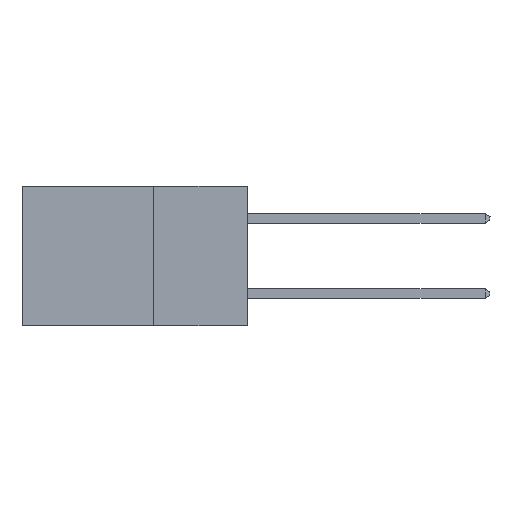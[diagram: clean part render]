
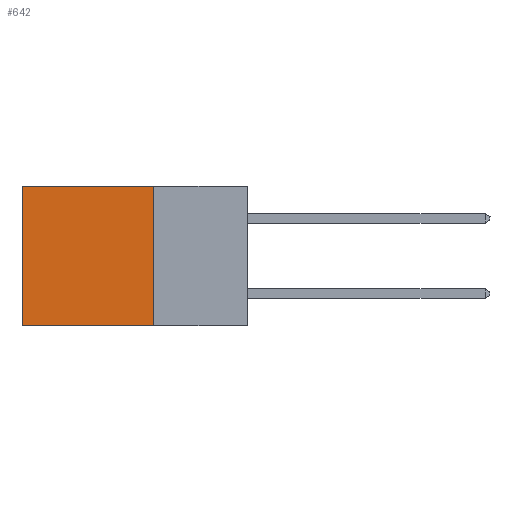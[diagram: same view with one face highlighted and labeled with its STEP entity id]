
A CAD part, left-side view. The second image highlights one B-rep face of the part: STEP entity #642.
In plain terms, the highlighted planar face has unit normal (-1, 0, 0).
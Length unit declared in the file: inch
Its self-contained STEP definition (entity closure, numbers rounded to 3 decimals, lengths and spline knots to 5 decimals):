
#642 = ADVANCED_FACE ( 'NONE', ( #13004 ), #6537, .F. ) ;
#854 = LINE ( 'NONE', #12288, #13545 ) ;
#1050 = ORIENTED_EDGE ( 'NONE', *, *, #10597, .T. ) ;
#1230 = LINE ( 'NONE', #1311, #15029 ) ;
#1311 = CARTESIAN_POINT ( 'NONE',  ( 0.2615, 0.6, -0.37 ) ) ;
#1510 = CARTESIAN_POINT ( 'NONE',  ( 0.2615, 0.25, -0.37 ) ) ;
#1747 = VECTOR ( 'NONE', #9764, 39.37008 ) ;
#2058 = CARTESIAN_POINT ( 'NONE',  ( 0.2615, 0.25, -0.37 ) ) ;
#2668 = VECTOR ( 'NONE', #13031, 39.37008 ) ;
#2673 = DIRECTION ( 'NONE',  ( 0., 0., -1. ) ) ;
#3038 = LINE ( 'NONE', #16051, #1747 ) ;
#3179 = EDGE_CURVE ( 'NONE', #6813, #14620, #854, .T. ) ;
#3225 = EDGE_CURVE ( 'NONE', #6813, #12833, #13723, .T. ) ;
#4881 = VERTEX_POINT ( 'NONE', #6152 ) ;
#5617 = AXIS2_PLACEMENT_3D ( 'NONE', #1510, #14443, #11566 ) ;
#6152 = CARTESIAN_POINT ( 'NONE',  ( 0.2615, 0.6, -0.37 ) ) ;
#6537 = PLANE ( 'NONE',  #5617 ) ;
#6813 = VERTEX_POINT ( 'NONE', #10483 ) ;
#7892 = ORIENTED_EDGE ( 'NONE', *, *, #3179, .T. ) ;
#9566 = ORIENTED_EDGE ( 'NONE', *, *, #11661, .F. ) ;
#9764 = DIRECTION ( 'NONE',  ( 0., 1., 0. ) ) ;
#9812 = DIRECTION ( 'NONE',  ( 0., 1., 0. ) ) ;
#10483 = CARTESIAN_POINT ( 'NONE',  ( 0.2615, 0.25, 0. ) ) ;
#10597 = EDGE_CURVE ( 'NONE', #14620, #4881, #1230, .T. ) ;
#11566 = DIRECTION ( 'NONE',  ( 0., 0., -1. ) ) ;
#11661 = EDGE_CURVE ( 'NONE', #12833, #4881, #3038, .T. ) ;
#11673 = EDGE_LOOP ( 'NONE', ( #1050, #9566, #12453, #7892 ) ) ;
#12288 = CARTESIAN_POINT ( 'NONE',  ( 0.2615, 0.25, 0. ) ) ;
#12453 = ORIENTED_EDGE ( 'NONE', *, *, #3225, .F. ) ;
#12595 = CARTESIAN_POINT ( 'NONE',  ( 0.2615, 0.25, -0.37 ) ) ;
#12833 = VERTEX_POINT ( 'NONE', #12595 ) ;
#13004 = FACE_OUTER_BOUND ( 'NONE', #11673, .T. ) ;
#13031 = DIRECTION ( 'NONE',  ( 0., 0., -1. ) ) ;
#13441 = CARTESIAN_POINT ( 'NONE',  ( 0.2615, 0.6, 0. ) ) ;
#13545 = VECTOR ( 'NONE', #9812, 39.37008 ) ;
#13723 = LINE ( 'NONE', #2058, #2668 ) ;
#14443 = DIRECTION ( 'NONE',  ( 1., 0., 0. ) ) ;
#14620 = VERTEX_POINT ( 'NONE', #13441 ) ;
#15029 = VECTOR ( 'NONE', #2673, 39.37008 ) ;
#16051 = CARTESIAN_POINT ( 'NONE',  ( 0.2615, 0.25, -0.37 ) ) ;
